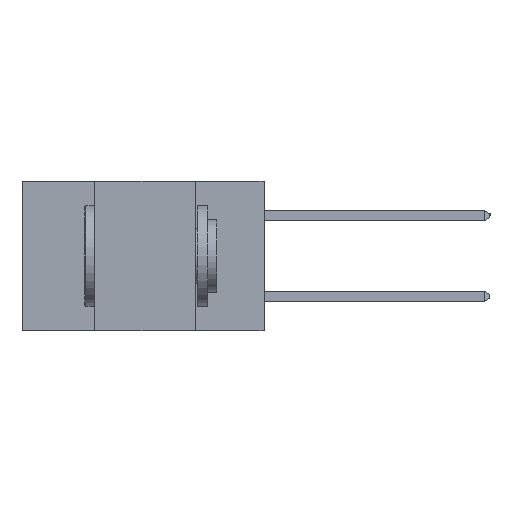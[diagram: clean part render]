
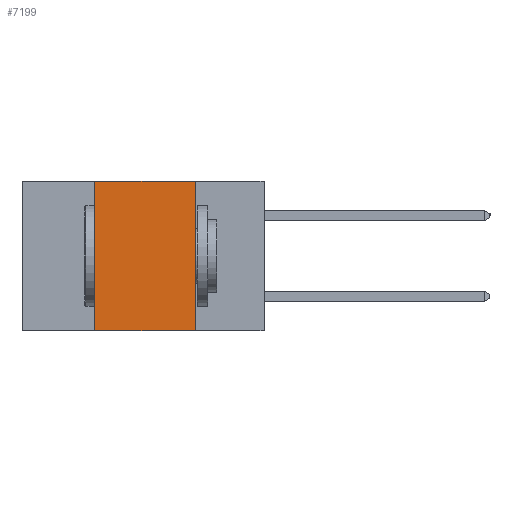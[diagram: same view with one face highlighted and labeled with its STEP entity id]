
A CAD part, left-side view. The second image highlights one B-rep face of the part: STEP entity #7199.
In plain terms, the highlighted planar face has unit normal (-1, 0, 0).
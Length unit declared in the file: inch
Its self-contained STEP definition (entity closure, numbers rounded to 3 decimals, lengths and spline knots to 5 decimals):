
#29 = CARTESIAN_POINT ( 'NONE',  ( 0., 0.42, -0.37 ) ) ;
#161 = CARTESIAN_POINT ( 'NONE',  ( 0., 0.42, -0.37 ) ) ;
#974 = FACE_OUTER_BOUND ( 'NONE', #19087, .T. ) ;
#1296 = EDGE_CURVE ( 'NONE', #21173, #12824, #9779, .T. ) ;
#1710 = CARTESIAN_POINT ( 'NONE',  ( 0., 0.42, 0. ) ) ;
#2048 = AXIS2_PLACEMENT_3D ( 'NONE', #12265, #2358, #10172 ) ;
#2358 = DIRECTION ( 'NONE',  ( 1., 0., 0. ) ) ;
#3110 = EDGE_CURVE ( 'NONE', #13416, #21173, #9866, .T. ) ;
#3235 = CARTESIAN_POINT ( 'NONE',  ( 0., 0.17, -0.37 ) ) ;
#4478 = VECTOR ( 'NONE', #7764, 39.37008 ) ;
#5621 = CARTESIAN_POINT ( 'NONE',  ( 0., 0.6, 0. ) ) ;
#6657 = CARTESIAN_POINT ( 'NONE',  ( 0., 0.17, -0.37 ) ) ;
#7091 = ORIENTED_EDGE ( 'NONE', *, *, #3110, .F. ) ;
#7199 = ADVANCED_FACE ( 'NONE', ( #974 ), #14147, .F. ) ;
#7764 = DIRECTION ( 'NONE',  ( 0., -1., 0. ) ) ;
#7851 = DIRECTION ( 'NONE',  ( 0., -1., 0. ) ) ;
#8562 = VERTEX_POINT ( 'NONE', #6657 ) ;
#9694 = EDGE_CURVE ( 'NONE', #13416, #8562, #19466, .T. ) ;
#9779 = LINE ( 'NONE', #5621, #4478 ) ;
#9866 = LINE ( 'NONE', #29, #20037 ) ;
#10172 = DIRECTION ( 'NONE',  ( 0., 0., -1. ) ) ;
#11131 = CARTESIAN_POINT ( 'NONE',  ( 0., 0.17, 0. ) ) ;
#12265 = CARTESIAN_POINT ( 'NONE',  ( 0., 0.6, 0. ) ) ;
#12824 = VERTEX_POINT ( 'NONE', #11131 ) ;
#13374 = CARTESIAN_POINT ( 'NONE',  ( 0., 0.6, -0.37 ) ) ;
#13416 = VERTEX_POINT ( 'NONE', #161 ) ;
#13585 = DIRECTION ( 'NONE',  ( 0., 0., 1. ) ) ;
#13907 = ORIENTED_EDGE ( 'NONE', *, *, #9694, .T. ) ;
#14015 = EDGE_CURVE ( 'NONE', #12824, #8562, #14633, .T. ) ;
#14147 = PLANE ( 'NONE',  #2048 ) ;
#14633 = LINE ( 'NONE', #3235, #16404 ) ;
#16404 = VECTOR ( 'NONE', #21873, 39.37008 ) ;
#18079 = ORIENTED_EDGE ( 'NONE', *, *, #1296, .F. ) ;
#18423 = ORIENTED_EDGE ( 'NONE', *, *, #14015, .F. ) ;
#19087 = EDGE_LOOP ( 'NONE', ( #18423, #18079, #7091, #13907 ) ) ;
#19466 = LINE ( 'NONE', #13374, #24551 ) ;
#20037 = VECTOR ( 'NONE', #13585, 39.37008 ) ;
#21173 = VERTEX_POINT ( 'NONE', #1710 ) ;
#21873 = DIRECTION ( 'NONE',  ( 0., 0., -1. ) ) ;
#24551 = VECTOR ( 'NONE', #7851, 39.37008 ) ;
